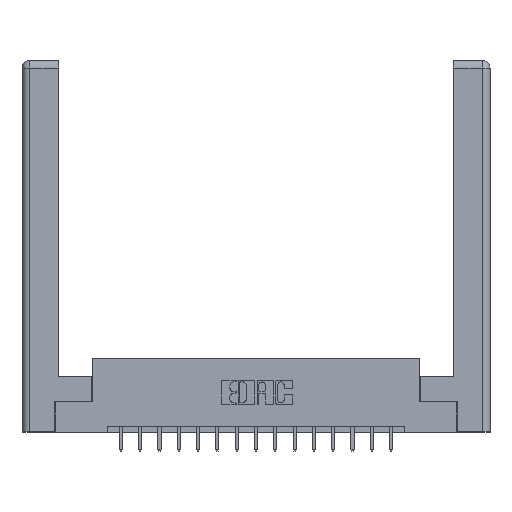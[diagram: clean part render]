
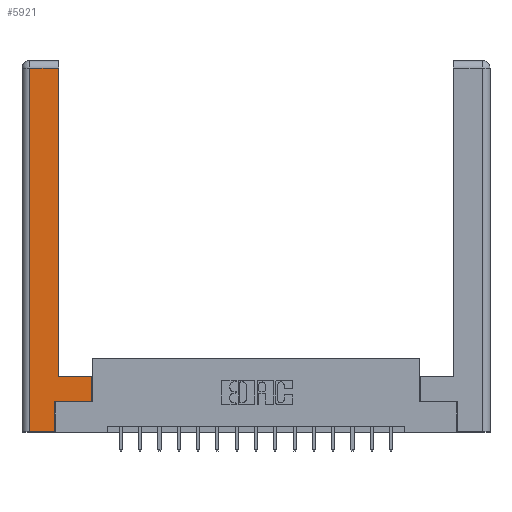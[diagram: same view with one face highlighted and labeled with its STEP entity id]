
A CAD part, top view. The second image highlights one B-rep face of the part: STEP entity #5921.
In plain terms, the highlighted planar face has unit normal (0, 0, 1).
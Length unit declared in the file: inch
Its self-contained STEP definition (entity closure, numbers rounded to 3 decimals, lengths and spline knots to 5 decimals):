
#37 = LINE ( 'NONE', #2570, #13806 ) ;
#265 = VERTEX_POINT ( 'NONE', #3651 ) ;
#422 = CARTESIAN_POINT ( 'NONE',  ( 0.0615, 0., 0. ) ) ;
#882 = VERTEX_POINT ( 'NONE', #1194 ) ;
#1125 = CARTESIAN_POINT ( 'NONE',  ( 0.295, 0.45, 0. ) ) ;
#1194 = CARTESIAN_POINT ( 'NONE',  ( 0.565, 0.45, 0. ) ) ;
#1299 = VECTOR ( 'NONE', #9768, 39.37008 ) ;
#1333 = CARTESIAN_POINT ( 'NONE',  ( 0.0615, 0., 0. ) ) ;
#1398 = CARTESIAN_POINT ( 'NONE',  ( 0.565, 0.245, 0. ) ) ;
#1411 = VECTOR ( 'NONE', #12151, 39.37008 ) ;
#1464 = CARTESIAN_POINT ( 'NONE',  ( 0.0615, 2.94, 0. ) ) ;
#1763 = CARTESIAN_POINT ( 'NONE',  ( 0.295, 3., 0. ) ) ;
#2163 = EDGE_CURVE ( 'NONE', #12267, #16472, #11098, .T. ) ;
#2274 = DIRECTION ( 'NONE',  ( 1., 0., 0. ) ) ;
#2570 = CARTESIAN_POINT ( 'NONE',  ( 0.265, 0., 0. ) ) ;
#2583 = ORIENTED_EDGE ( 'NONE', *, *, #10209, .T. ) ;
#2642 = LINE ( 'NONE', #1464, #17052 ) ;
#2975 = CARTESIAN_POINT ( 'NONE',  ( 0., 0., 0. ) ) ;
#3041 = DIRECTION ( 'NONE',  ( -1., 0., 0. ) ) ;
#3089 = ORIENTED_EDGE ( 'NONE', *, *, #12208, .T. ) ;
#3651 = CARTESIAN_POINT ( 'NONE',  ( 0.0615, 2.94, 0. ) ) ;
#4113 = EDGE_CURVE ( 'NONE', #10138, #12267, #37, .T. ) ;
#5093 = LINE ( 'NONE', #1398, #7502 ) ;
#5735 = LINE ( 'NONE', #13256, #14791 ) ;
#5921 = ADVANCED_FACE ( 'NONE', ( #15231 ), #16573, .F. ) ;
#6522 = VECTOR ( 'NONE', #10125, 39.37008 ) ;
#7502 = VECTOR ( 'NONE', #2274, 39.37008 ) ;
#7508 = DIRECTION ( 'NONE',  ( 0., 1., 0. ) ) ;
#8085 = DIRECTION ( 'NONE',  ( 0., 1., 0. ) ) ;
#8235 = EDGE_CURVE ( 'NONE', #11410, #15760, #9927, .T. ) ;
#9543 = CARTESIAN_POINT ( 'NONE',  ( 0.265, 0.245, 0. ) ) ;
#9643 = CARTESIAN_POINT ( 'NONE',  ( 0.565, 0.245, 0. ) ) ;
#9768 = DIRECTION ( 'NONE',  ( 0., 1., 0. ) ) ;
#9927 = LINE ( 'NONE', #1763, #1299 ) ;
#10125 = DIRECTION ( 'NONE',  ( 0., -1., 0. ) ) ;
#10138 = VERTEX_POINT ( 'NONE', #1333 ) ;
#10163 = VERTEX_POINT ( 'NONE', #9643 ) ;
#10209 = EDGE_CURVE ( 'NONE', #16472, #10163, #5093, .T. ) ;
#10781 = EDGE_CURVE ( 'NONE', #882, #11410, #16463, .T. ) ;
#11068 = DIRECTION ( 'NONE',  ( 0., 0., -1. ) ) ;
#11092 = DIRECTION ( 'NONE',  ( -1., 0., 0. ) ) ;
#11098 = LINE ( 'NONE', #13524, #16667 ) ;
#11309 = ORIENTED_EDGE ( 'NONE', *, *, #16005, .T. ) ;
#11410 = VERTEX_POINT ( 'NONE', #1125 ) ;
#11440 = AXIS2_PLACEMENT_3D ( 'NONE', #2975, #11068, #3041 ) ;
#11647 = ORIENTED_EDGE ( 'NONE', *, *, #4113, .T. ) ;
#11703 = ORIENTED_EDGE ( 'NONE', *, *, #8235, .T. ) ;
#12151 = DIRECTION ( 'NONE',  ( -1., 0., 0. ) ) ;
#12200 = DIRECTION ( 'NONE',  ( 1., 0., 0. ) ) ;
#12208 = EDGE_CURVE ( 'NONE', #15760, #265, #2642, .T. ) ;
#12215 = CARTESIAN_POINT ( 'NONE',  ( 0.295, 2.94, 0. ) ) ;
#12267 = VERTEX_POINT ( 'NONE', #14213 ) ;
#13256 = CARTESIAN_POINT ( 'NONE',  ( 0.565, 0.45, 0. ) ) ;
#13418 = ORIENTED_EDGE ( 'NONE', *, *, #2163, .T. ) ;
#13524 = CARTESIAN_POINT ( 'NONE',  ( 0.265, 0.245, 0. ) ) ;
#13566 = EDGE_CURVE ( 'NONE', #10163, #882, #5735, .T. ) ;
#13806 = VECTOR ( 'NONE', #12200, 39.37008 ) ;
#14213 = CARTESIAN_POINT ( 'NONE',  ( 0.265, 0., 0. ) ) ;
#14791 = VECTOR ( 'NONE', #7508, 39.37008 ) ;
#15231 = FACE_OUTER_BOUND ( 'NONE', #17665, .T. ) ;
#15733 = LINE ( 'NONE', #422, #6522 ) ;
#15760 = VERTEX_POINT ( 'NONE', #12215 ) ;
#16005 = EDGE_CURVE ( 'NONE', #265, #10138, #15733, .T. ) ;
#16279 = CARTESIAN_POINT ( 'NONE',  ( 0.295, 0.45, 0. ) ) ;
#16463 = LINE ( 'NONE', #16279, #1411 ) ;
#16472 = VERTEX_POINT ( 'NONE', #9543 ) ;
#16552 = ORIENTED_EDGE ( 'NONE', *, *, #13566, .T. ) ;
#16573 = PLANE ( 'NONE',  #11440 ) ;
#16624 = ORIENTED_EDGE ( 'NONE', *, *, #10781, .T. ) ;
#16667 = VECTOR ( 'NONE', #8085, 39.37008 ) ;
#17052 = VECTOR ( 'NONE', #11092, 39.37008 ) ;
#17665 = EDGE_LOOP ( 'NONE', ( #11703, #3089, #11309, #11647, #13418, #2583, #16552, #16624 ) ) ;
